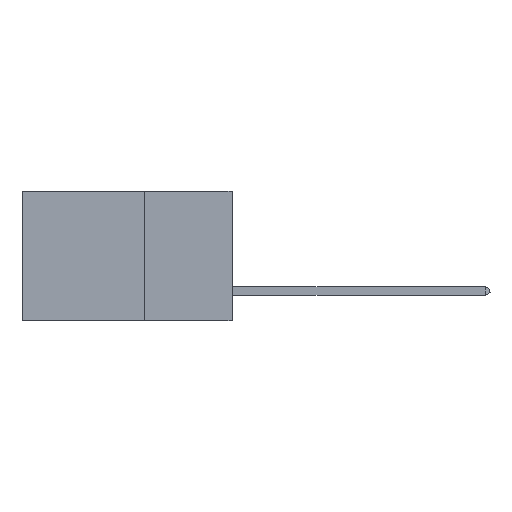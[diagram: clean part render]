
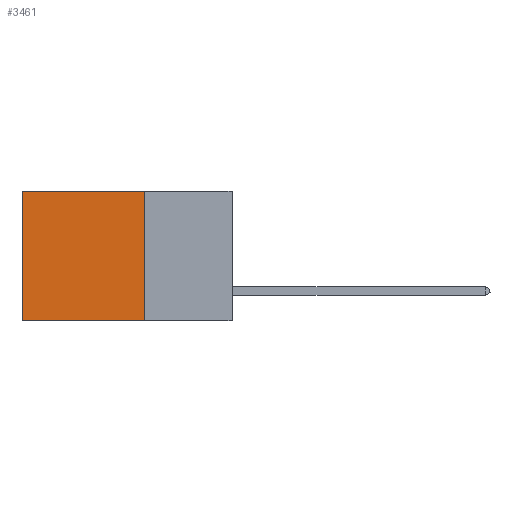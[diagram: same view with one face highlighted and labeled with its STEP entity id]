
A CAD part, left-side view. The second image highlights one B-rep face of the part: STEP entity #3461.
In plain terms, the highlighted planar face has unit normal (-1, 0, 0).
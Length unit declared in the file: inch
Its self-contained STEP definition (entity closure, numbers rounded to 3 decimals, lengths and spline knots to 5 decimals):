
#79 = CARTESIAN_POINT ( 'NONE',  ( 0.2875, 0.6, 0. ) ) ;
#190 = CARTESIAN_POINT ( 'NONE',  ( 0.2875, 0.25, -0.37 ) ) ;
#2755 = VECTOR ( 'NONE', #4423, 39.37008 ) ;
#2846 = ORIENTED_EDGE ( 'NONE', *, *, #20853, .F. ) ;
#3461 = ADVANCED_FACE ( 'NONE', ( #26278 ), #19105, .F. ) ;
#4423 = DIRECTION ( 'NONE',  ( 0., 0., -1. ) ) ;
#4477 = VECTOR ( 'NONE', #15142, 39.37008 ) ;
#5349 = AXIS2_PLACEMENT_3D ( 'NONE', #25493, #8547, #12669 ) ;
#5696 = LINE ( 'NONE', #21552, #8109 ) ;
#6285 = CARTESIAN_POINT ( 'NONE',  ( 0.2875, 0.6, -0.37 ) ) ;
#7294 = DIRECTION ( 'NONE',  ( 0., 1., 0. ) ) ;
#7569 = VERTEX_POINT ( 'NONE', #8618 ) ;
#7868 = LINE ( 'NONE', #79, #2755 ) ;
#7920 = ORIENTED_EDGE ( 'NONE', *, *, #16270, .F. ) ;
#8109 = VECTOR ( 'NONE', #13028, 39.37008 ) ;
#8547 = DIRECTION ( 'NONE',  ( 1., 0., 0. ) ) ;
#8618 = CARTESIAN_POINT ( 'NONE',  ( 0.2875, 0.25, 0. ) ) ;
#8650 = EDGE_CURVE ( 'NONE', #7569, #14650, #5696, .T. ) ;
#11561 = VERTEX_POINT ( 'NONE', #19911 ) ;
#12669 = DIRECTION ( 'NONE',  ( 0., 0., -1. ) ) ;
#12810 = CARTESIAN_POINT ( 'NONE',  ( 0.2875, 0.25, 0. ) ) ;
#13028 = DIRECTION ( 'NONE',  ( 0., 1., 0. ) ) ;
#14650 = VERTEX_POINT ( 'NONE', #23858 ) ;
#15142 = DIRECTION ( 'NONE',  ( 0., 0., -1. ) ) ;
#16270 = EDGE_CURVE ( 'NONE', #11561, #25828, #27731, .T. ) ;
#19105 = PLANE ( 'NONE',  #5349 ) ;
#19568 = EDGE_LOOP ( 'NONE', ( #25726, #7920, #2846, #23652 ) ) ;
#19675 = EDGE_CURVE ( 'NONE', #14650, #25828, #7868, .T. ) ;
#19911 = CARTESIAN_POINT ( 'NONE',  ( 0.2875, 0.25, -0.37 ) ) ;
#20853 = EDGE_CURVE ( 'NONE', #7569, #11561, #27308, .T. ) ;
#21552 = CARTESIAN_POINT ( 'NONE',  ( 0.2875, 0.25, 0. ) ) ;
#23025 = VECTOR ( 'NONE', #7294, 39.37008 ) ;
#23652 = ORIENTED_EDGE ( 'NONE', *, *, #8650, .T. ) ;
#23858 = CARTESIAN_POINT ( 'NONE',  ( 0.2875, 0.6, 0. ) ) ;
#25493 = CARTESIAN_POINT ( 'NONE',  ( 0.2875, 0.25, 0. ) ) ;
#25726 = ORIENTED_EDGE ( 'NONE', *, *, #19675, .T. ) ;
#25828 = VERTEX_POINT ( 'NONE', #6285 ) ;
#26278 = FACE_OUTER_BOUND ( 'NONE', #19568, .T. ) ;
#27308 = LINE ( 'NONE', #12810, #4477 ) ;
#27731 = LINE ( 'NONE', #190, #23025 ) ;
